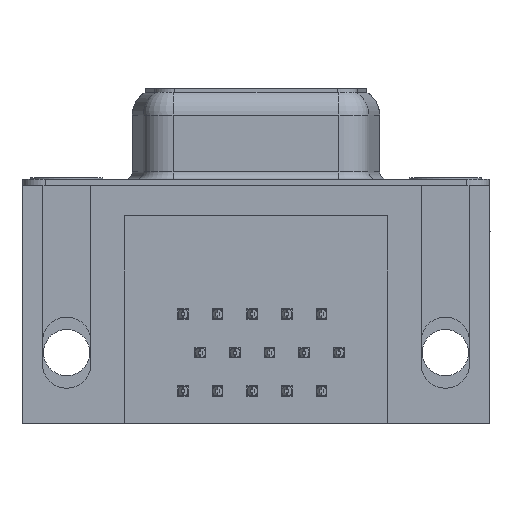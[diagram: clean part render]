
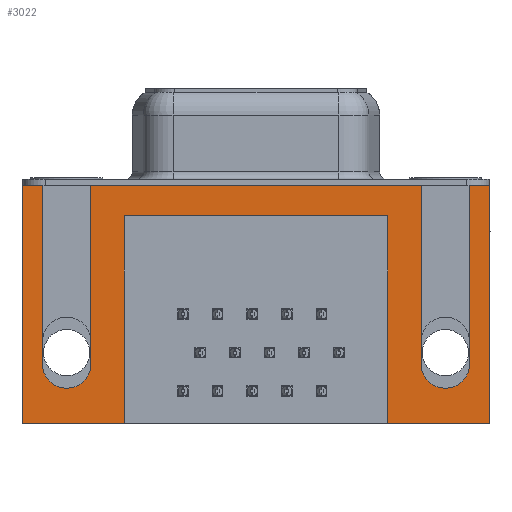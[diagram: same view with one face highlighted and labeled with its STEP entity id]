
A CAD part, front view. The second image highlights one B-rep face of the part: STEP entity #3022.
In plain terms, the highlighted planar face has unit normal (0, -1, 0).
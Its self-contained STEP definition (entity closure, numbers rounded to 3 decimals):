
#263 = ORIENTED_EDGE ( 'NONE', *, *, #24066, .F. ) ;
#579 = CARTESIAN_POINT ( 'NONE',  ( -2.91, -6.275, 0. ) ) ;
#1470 = LINE ( 'NONE', #34164, #22087 ) ;
#1696 = FACE_OUTER_BOUND ( 'NONE', #28786, .T. ) ;
#1765 = EDGE_CURVE ( 'NONE', #19535, #4569, #19395, .T. ) ;
#1976 = VECTOR ( 'NONE', #5115, 1000. ) ;
#2701 = VERTEX_POINT ( 'NONE', #32678 ) ;
#2813 = LINE ( 'NONE', #7810, #1976 ) ;
#2867 = EDGE_CURVE ( 'NONE', #34114, #33128, #33782, .T. ) ;
#2927 = ORIENTED_EDGE ( 'NONE', *, *, #16333, .F. ) ;
#3022 = ADVANCED_FACE ( 'NONE', ( #1696 ), #31679, .T. ) ;
#3186 = EDGE_CURVE ( 'NONE', #20488, #30133, #11669, .T. ) ;
#3365 = ORIENTED_EDGE ( 'NONE', *, *, #9977, .F. ) ;
#4253 = ORIENTED_EDGE ( 'NONE', *, *, #9333, .T. ) ;
#4276 = EDGE_CURVE ( 'NONE', #8992, #7116, #23087, .T. ) ;
#4373 = CARTESIAN_POINT ( 'NONE',  ( 21.2, -6.275, -2. ) ) ;
#4479 = VECTOR ( 'NONE', #24110, 1000. ) ;
#4569 = VERTEX_POINT ( 'NONE', #24810 ) ;
#4759 = VERTEX_POINT ( 'NONE', #22903 ) ;
#4777 = DIRECTION ( 'NONE',  ( 0., 0., 1. ) ) ;
#4927 = AXIS2_PLACEMENT_3D ( 'NONE', #23651, #7438, #26396 ) ;
#5115 = DIRECTION ( 'NONE',  ( 0., 0., -1. ) ) ;
#5201 = CARTESIAN_POINT ( 'NONE',  ( 3.79, -6.275, -2. ) ) ;
#5347 = CARTESIAN_POINT ( 'NONE',  ( 3.79, -6.275, -2. ) ) ;
#5350 = CARTESIAN_POINT ( 'NONE',  ( -1.6, -6.275, 0. ) ) ;
#5746 = LINE ( 'NONE', #21954, #20111 ) ;
#5762 = DIRECTION ( 'NONE',  ( 0., 0., -1. ) ) ;
#7079 = EDGE_CURVE ( 'NONE', #7116, #2701, #2813, .T. ) ;
#7116 = VERTEX_POINT ( 'NONE', #5350 ) ;
#7152 = CARTESIAN_POINT ( 'NONE',  ( -2.91, -6.275, 0. ) ) ;
#7299 = DIRECTION ( 'NONE',  ( 0., 0., 1. ) ) ;
#7400 = DIRECTION ( 'NONE',  ( 0., 0., -1. ) ) ;
#7438 = DIRECTION ( 'NONE',  ( 0., -1., 0. ) ) ;
#7810 = CARTESIAN_POINT ( 'NONE',  ( -1.6, -6.275, 0. ) ) ;
#8527 = CARTESIAN_POINT ( 'NONE',  ( 23.39, -6.275, -11.78 ) ) ;
#8992 = VERTEX_POINT ( 'NONE', #24334 ) ;
#9333 = EDGE_CURVE ( 'NONE', #19405, #34494, #1470, .T. ) ;
#9531 = EDGE_CURVE ( 'NONE', #19405, #15790, #32243, .T. ) ;
#9977 = EDGE_CURVE ( 'NONE', #33128, #16375, #21168, .T. ) ;
#10108 = VECTOR ( 'NONE', #14856, 1000. ) ;
#10493 = AXIS2_PLACEMENT_3D ( 'NONE', #18124, #23618, #7400 ) ;
#10521 = CARTESIAN_POINT ( 'NONE',  ( 27.9, -6.275, -15.7 ) ) ;
#10524 = LINE ( 'NONE', #23035, #11391 ) ;
#10694 = CARTESIAN_POINT ( 'NONE',  ( -2.91, -6.275, 0. ) ) ;
#11391 = VECTOR ( 'NONE', #7299, 1000. ) ;
#11669 = LINE ( 'NONE', #579, #32483 ) ;
#12443 = EDGE_CURVE ( 'NONE', #16375, #34494, #13434, .T. ) ;
#12696 = LINE ( 'NONE', #22720, #26311 ) ;
#13165 = VECTOR ( 'NONE', #20510, 1000. ) ;
#13184 = ORIENTED_EDGE ( 'NONE', *, *, #28867, .F. ) ;
#13410 = DIRECTION ( 'NONE',  ( 1., 0., 0. ) ) ;
#13434 = LINE ( 'NONE', #7152, #34261 ) ;
#13845 = DIRECTION ( 'NONE',  ( 1., 0., 0. ) ) ;
#14051 = CARTESIAN_POINT ( 'NONE',  ( 27.9, -6.275, -15.7 ) ) ;
#14124 = CARTESIAN_POINT ( 'NONE',  ( 1.6, -6.275, 0. ) ) ;
#14469 = DIRECTION ( 'NONE',  ( 0., -1., 0. ) ) ;
#14856 = DIRECTION ( 'NONE',  ( -1., 0., 0. ) ) ;
#14914 = CARTESIAN_POINT ( 'NONE',  ( 3.79, -6.275, -15.7 ) ) ;
#14961 = EDGE_CURVE ( 'NONE', #15790, #4759, #34843, .T. ) ;
#15154 = DIRECTION ( 'NONE',  ( 0., 0., 1. ) ) ;
#15790 = VERTEX_POINT ( 'NONE', #30434 ) ;
#15835 = VECTOR ( 'NONE', #13410, 1000. ) ;
#15882 = EDGE_CURVE ( 'NONE', #4569, #8992, #12696, .T. ) ;
#15920 = ORIENTED_EDGE ( 'NONE', *, *, #7079, .F. ) ;
#16333 = EDGE_CURVE ( 'NONE', #2701, #18553, #16910, .T. ) ;
#16375 = VERTEX_POINT ( 'NONE', #32301 ) ;
#16554 = DIRECTION ( 'NONE',  ( -1., 0., 0. ) ) ;
#16682 = ORIENTED_EDGE ( 'NONE', *, *, #17913, .F. ) ;
#16910 = CIRCLE ( 'NONE', #4927, 1.6 ) ;
#16932 = VECTOR ( 'NONE', #24176, 1000. ) ;
#17583 = ORIENTED_EDGE ( 'NONE', *, *, #31349, .F. ) ;
#17696 = CARTESIAN_POINT ( 'NONE',  ( 1.6, -6.275, -11.78 ) ) ;
#17913 = EDGE_CURVE ( 'NONE', #18553, #20488, #10524, .T. ) ;
#18124 = CARTESIAN_POINT ( 'NONE',  ( -2.91, -6.275, -2.5 ) ) ;
#18135 = ORIENTED_EDGE ( 'NONE', *, *, #2867, .F. ) ;
#18553 = VERTEX_POINT ( 'NONE', #17696 ) ;
#19395 = LINE ( 'NONE', #14051, #20248 ) ;
#19405 = VERTEX_POINT ( 'NONE', #25536 ) ;
#19535 = VERTEX_POINT ( 'NONE', #14914 ) ;
#20111 = VECTOR ( 'NONE', #5762, 1000. ) ;
#20248 = VECTOR ( 'NONE', #16554, 1000. ) ;
#20274 = AXIS2_PLACEMENT_3D ( 'NONE', #30761, #14469, #33502 ) ;
#20327 = VECTOR ( 'NONE', #4777, 1000. ) ;
#20488 = VERTEX_POINT ( 'NONE', #14124 ) ;
#20510 = DIRECTION ( 'NONE',  ( 0., 0., 1. ) ) ;
#20927 = CARTESIAN_POINT ( 'NONE',  ( 26.59, -6.275, 0. ) ) ;
#21168 = LINE ( 'NONE', #20927, #20327 ) ;
#21603 = CARTESIAN_POINT ( 'NONE',  ( 26.59, -6.275, -11.78 ) ) ;
#21691 = ORIENTED_EDGE ( 'NONE', *, *, #1765, .F. ) ;
#21954 = CARTESIAN_POINT ( 'NONE',  ( 23.39, -6.275, 0. ) ) ;
#22087 = VECTOR ( 'NONE', #15154, 1000. ) ;
#22720 = CARTESIAN_POINT ( 'NONE',  ( -2.91, -6.275, -2.5 ) ) ;
#22903 = CARTESIAN_POINT ( 'NONE',  ( 21.2, -6.275, -2. ) ) ;
#23035 = CARTESIAN_POINT ( 'NONE',  ( 1.6, -6.275, 0. ) ) ;
#23087 = LINE ( 'NONE', #10694, #15835 ) ;
#23618 = DIRECTION ( 'NONE',  ( 0., -1., 0. ) ) ;
#23651 = CARTESIAN_POINT ( 'NONE',  ( 0., -6.275, -11.78 ) ) ;
#23716 = LINE ( 'NONE', #33874, #10108 ) ;
#24066 = EDGE_CURVE ( 'NONE', #4759, #34024, #23716, .T. ) ;
#24110 = DIRECTION ( 'NONE',  ( 0., 0., -1. ) ) ;
#24176 = DIRECTION ( 'NONE',  ( -1., 0., 0. ) ) ;
#24334 = CARTESIAN_POINT ( 'NONE',  ( -2.91, -6.275, 0. ) ) ;
#24622 = ORIENTED_EDGE ( 'NONE', *, *, #15882, .F. ) ;
#24810 = CARTESIAN_POINT ( 'NONE',  ( -2.91, -6.275, -15.7 ) ) ;
#25209 = LINE ( 'NONE', #5201, #4479 ) ;
#25458 = DIRECTION ( 'NONE',  ( 0., 0., 1. ) ) ;
#25536 = CARTESIAN_POINT ( 'NONE',  ( 27.9, -6.275, -15.7 ) ) ;
#25968 = ORIENTED_EDGE ( 'NONE', *, *, #4276, .F. ) ;
#26311 = VECTOR ( 'NONE', #25458, 1000. ) ;
#26396 = DIRECTION ( 'NONE',  ( 1., 0., 0. ) ) ;
#27960 = ORIENTED_EDGE ( 'NONE', *, *, #14961, .F. ) ;
#28617 = CARTESIAN_POINT ( 'NONE',  ( 23.39, -6.275, 0. ) ) ;
#28786 = EDGE_LOOP ( 'NONE', ( #3365, #18135, #13184, #32302, #16682, #2927, #15920, #25968, #24622, #21691, #17583, #263, #27960, #34586, #4253, #28948 ) ) ;
#28867 = EDGE_CURVE ( 'NONE', #30133, #34114, #5746, .T. ) ;
#28933 = DIRECTION ( 'NONE',  ( 1., 0., 0. ) ) ;
#28948 = ORIENTED_EDGE ( 'NONE', *, *, #12443, .F. ) ;
#30133 = VERTEX_POINT ( 'NONE', #28617 ) ;
#30434 = CARTESIAN_POINT ( 'NONE',  ( 21.2, -6.275, -15.7 ) ) ;
#30761 = CARTESIAN_POINT ( 'NONE',  ( 24.99, -6.275, -11.78 ) ) ;
#31349 = EDGE_CURVE ( 'NONE', #34024, #19535, #25209, .T. ) ;
#31679 = PLANE ( 'NONE',  #10493 ) ;
#31812 = CARTESIAN_POINT ( 'NONE',  ( 27.9, -6.275, 0. ) ) ;
#32243 = LINE ( 'NONE', #10521, #16932 ) ;
#32301 = CARTESIAN_POINT ( 'NONE',  ( 26.59, -6.275, 0. ) ) ;
#32302 = ORIENTED_EDGE ( 'NONE', *, *, #3186, .F. ) ;
#32483 = VECTOR ( 'NONE', #13845, 1000. ) ;
#32678 = CARTESIAN_POINT ( 'NONE',  ( -1.6, -6.275, -11.78 ) ) ;
#33128 = VERTEX_POINT ( 'NONE', #21603 ) ;
#33502 = DIRECTION ( 'NONE',  ( -1., 0., 0. ) ) ;
#33782 = CIRCLE ( 'NONE', #20274, 1.6 ) ;
#33874 = CARTESIAN_POINT ( 'NONE',  ( 3.79, -6.275, -2. ) ) ;
#34024 = VERTEX_POINT ( 'NONE', #5347 ) ;
#34114 = VERTEX_POINT ( 'NONE', #8527 ) ;
#34164 = CARTESIAN_POINT ( 'NONE',  ( 27.9, -6.275, -2.5 ) ) ;
#34261 = VECTOR ( 'NONE', #28933, 1000. ) ;
#34494 = VERTEX_POINT ( 'NONE', #31812 ) ;
#34586 = ORIENTED_EDGE ( 'NONE', *, *, #9531, .F. ) ;
#34843 = LINE ( 'NONE', #4373, #13165 ) ;
